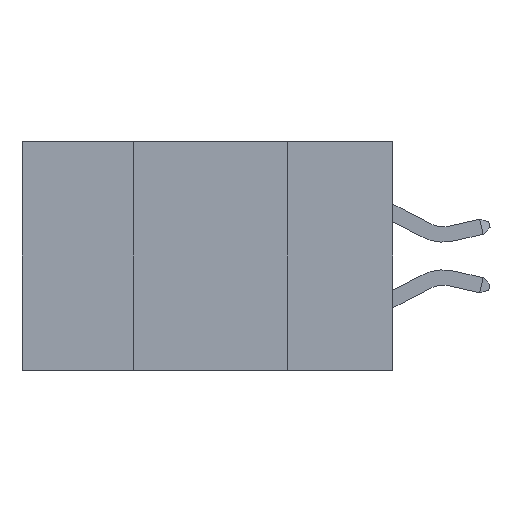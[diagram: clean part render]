
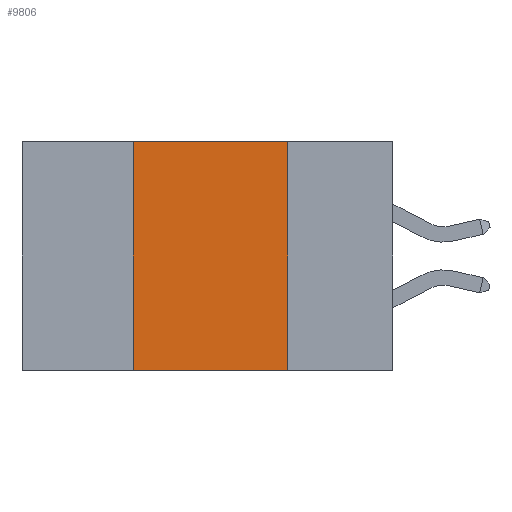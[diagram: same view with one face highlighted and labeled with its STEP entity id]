
A CAD part, left-side view. The second image highlights one B-rep face of the part: STEP entity #9806.
In plain terms, the highlighted planar face has unit normal (-1, 0, 0).
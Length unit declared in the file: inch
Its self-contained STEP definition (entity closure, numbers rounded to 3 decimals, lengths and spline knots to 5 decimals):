
#443 = CARTESIAN_POINT ( 'NONE',  ( 0., 0.17, 0. ) ) ;
#452 = DIRECTION ( 'NONE',  ( 1., 0., 0. ) ) ;
#547 = EDGE_CURVE ( 'NONE', #2620, #8729, #8102, .T. ) ;
#578 = EDGE_CURVE ( 'NONE', #7389, #7760, #7322, .T. ) ;
#1404 = EDGE_LOOP ( 'NONE', ( #9374, #9112, #8783, #7528 ) ) ;
#2003 = CARTESIAN_POINT ( 'NONE',  ( 0., 0.6, 0. ) ) ;
#2291 = CARTESIAN_POINT ( 'NONE',  ( 0., 0.17, -0.37 ) ) ;
#2620 = VERTEX_POINT ( 'NONE', #9791 ) ;
#2661 = CARTESIAN_POINT ( 'NONE',  ( 0., 0.6, -0.37 ) ) ;
#2885 = VECTOR ( 'NONE', #5427, 39.37008 ) ;
#2933 = DIRECTION ( 'NONE',  ( 0., -1., 0. ) ) ;
#3101 = LINE ( 'NONE', #2661, #7516 ) ;
#4394 = AXIS2_PLACEMENT_3D ( 'NONE', #10034, #452, #6691 ) ;
#5427 = DIRECTION ( 'NONE',  ( 0., 0., 1. ) ) ;
#6556 = CARTESIAN_POINT ( 'NONE',  ( 0., 0.17, 0. ) ) ;
#6691 = DIRECTION ( 'NONE',  ( 0., 0., -1. ) ) ;
#7092 = DIRECTION ( 'NONE',  ( 0., -1., 0. ) ) ;
#7322 = LINE ( 'NONE', #6556, #9271 ) ;
#7389 = VERTEX_POINT ( 'NONE', #443 ) ;
#7411 = DIRECTION ( 'NONE',  ( 0., 0., -1. ) ) ;
#7516 = VECTOR ( 'NONE', #7092, 39.37008 ) ;
#7528 = ORIENTED_EDGE ( 'NONE', *, *, #8452, .T. ) ;
#7760 = VERTEX_POINT ( 'NONE', #2291 ) ;
#7835 = VECTOR ( 'NONE', #2933, 39.37008 ) ;
#8102 = LINE ( 'NONE', #8217, #2885 ) ;
#8112 = LINE ( 'NONE', #2003, #7835 ) ;
#8217 = CARTESIAN_POINT ( 'NONE',  ( 0., 0.42, 0. ) ) ;
#8452 = EDGE_CURVE ( 'NONE', #2620, #7760, #3101, .T. ) ;
#8677 = FACE_OUTER_BOUND ( 'NONE', #1404, .T. ) ;
#8729 = VERTEX_POINT ( 'NONE', #10785 ) ;
#8783 = ORIENTED_EDGE ( 'NONE', *, *, #547, .F. ) ;
#9112 = ORIENTED_EDGE ( 'NONE', *, *, #11226, .F. ) ;
#9271 = VECTOR ( 'NONE', #7411, 39.37008 ) ;
#9374 = ORIENTED_EDGE ( 'NONE', *, *, #578, .F. ) ;
#9791 = CARTESIAN_POINT ( 'NONE',  ( 0., 0.42, -0.37 ) ) ;
#9806 = ADVANCED_FACE ( 'NONE', ( #8677 ), #10868, .F. ) ;
#10034 = CARTESIAN_POINT ( 'NONE',  ( 0., 0.6, 0. ) ) ;
#10785 = CARTESIAN_POINT ( 'NONE',  ( 0., 0.42, 0. ) ) ;
#10868 = PLANE ( 'NONE',  #4394 ) ;
#11226 = EDGE_CURVE ( 'NONE', #8729, #7389, #8112, .T. ) ;
